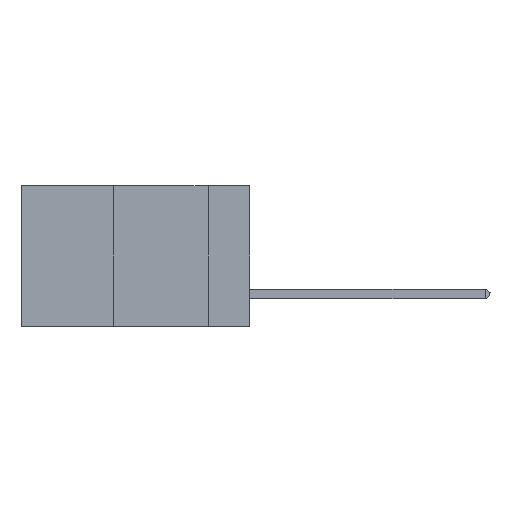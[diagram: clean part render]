
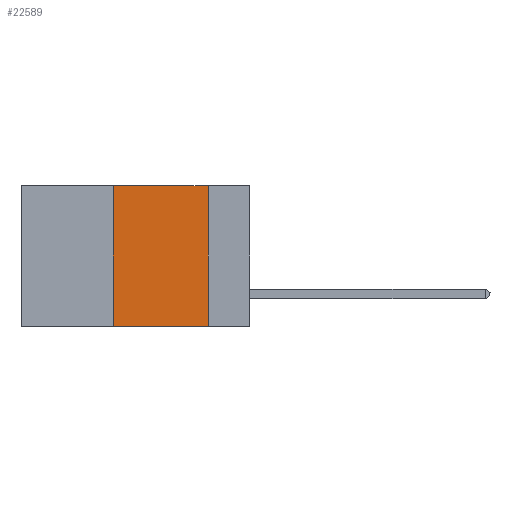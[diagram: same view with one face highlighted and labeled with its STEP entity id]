
A CAD part, left-side view. The second image highlights one B-rep face of the part: STEP entity #22589.
In plain terms, the highlighted planar face has unit normal (-1, 0, 0).
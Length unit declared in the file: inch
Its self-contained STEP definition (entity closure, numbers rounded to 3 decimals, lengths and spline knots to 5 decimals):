
#1675 = VECTOR ( 'NONE', #5629, 39.37008 ) ;
#1696 = CARTESIAN_POINT ( 'NONE',  ( 0., 0.11, -0.37 ) ) ;
#4235 = CARTESIAN_POINT ( 'NONE',  ( 0., 0.36, 0. ) ) ;
#4536 = ORIENTED_EDGE ( 'NONE', *, *, #12019, .F. ) ;
#5629 = DIRECTION ( 'NONE',  ( 0., -1., 0. ) ) ;
#7610 = EDGE_CURVE ( 'NONE', #26523, #25541, #21396, .T. ) ;
#7638 = PLANE ( 'NONE',  #21663 ) ;
#7849 = LINE ( 'NONE', #4235, #26716 ) ;
#8857 = VERTEX_POINT ( 'NONE', #19493 ) ;
#10458 = DIRECTION ( 'NONE',  ( 0., -1., 0. ) ) ;
#12019 = EDGE_CURVE ( 'NONE', #8857, #15772, #29844, .T. ) ;
#12840 = DIRECTION ( 'NONE',  ( 0., 0., 1. ) ) ;
#13014 = DIRECTION ( 'NONE',  ( 1., 0., 0. ) ) ;
#13338 = CARTESIAN_POINT ( 'NONE',  ( 0., 0.6, 0. ) ) ;
#15363 = CARTESIAN_POINT ( 'NONE',  ( 0., 0.36, -0.37 ) ) ;
#15772 = VERTEX_POINT ( 'NONE', #19015 ) ;
#16825 = VECTOR ( 'NONE', #27170, 39.37008 ) ;
#18129 = LINE ( 'NONE', #31957, #16825 ) ;
#19015 = CARTESIAN_POINT ( 'NONE',  ( 0., 0.11, 0. ) ) ;
#19493 = CARTESIAN_POINT ( 'NONE',  ( 0., 0.36, 0. ) ) ;
#21396 = LINE ( 'NONE', #31970, #1675 ) ;
#21663 = AXIS2_PLACEMENT_3D ( 'NONE', #29396, #13014, #34906 ) ;
#22486 = VECTOR ( 'NONE', #10458, 39.37008 ) ;
#22589 = ADVANCED_FACE ( 'NONE', ( #28184 ), #7638, .F. ) ;
#24271 = ORIENTED_EDGE ( 'NONE', *, *, #31089, .F. ) ;
#25541 = VERTEX_POINT ( 'NONE', #1696 ) ;
#26523 = VERTEX_POINT ( 'NONE', #15363 ) ;
#26716 = VECTOR ( 'NONE', #12840, 39.37008 ) ;
#27170 = DIRECTION ( 'NONE',  ( 0., 0., -1. ) ) ;
#28184 = FACE_OUTER_BOUND ( 'NONE', #30973, .T. ) ;
#28233 = ORIENTED_EDGE ( 'NONE', *, *, #30755, .F. ) ;
#29396 = CARTESIAN_POINT ( 'NONE',  ( 0., 0.6, 0. ) ) ;
#29844 = LINE ( 'NONE', #13338, #22486 ) ;
#30755 = EDGE_CURVE ( 'NONE', #15772, #25541, #18129, .T. ) ;
#30973 = EDGE_LOOP ( 'NONE', ( #28233, #4536, #24271, #34274 ) ) ;
#31089 = EDGE_CURVE ( 'NONE', #26523, #8857, #7849, .T. ) ;
#31957 = CARTESIAN_POINT ( 'NONE',  ( 0., 0.11, 0. ) ) ;
#31970 = CARTESIAN_POINT ( 'NONE',  ( 0., 0.6, -0.37 ) ) ;
#34274 = ORIENTED_EDGE ( 'NONE', *, *, #7610, .T. ) ;
#34906 = DIRECTION ( 'NONE',  ( 0., 0., -1. ) ) ;
